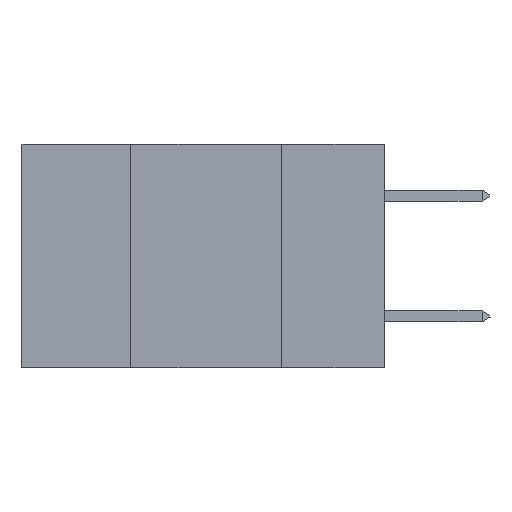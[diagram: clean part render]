
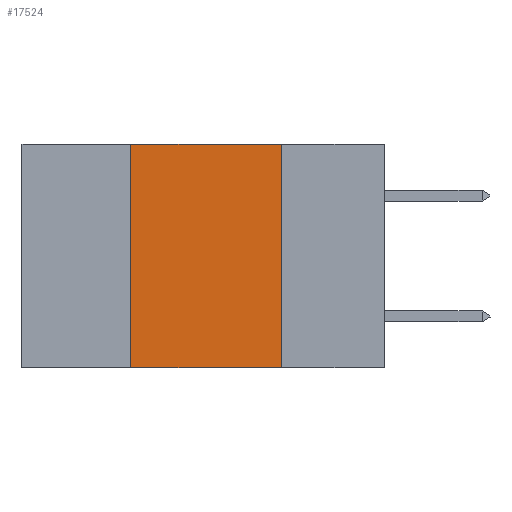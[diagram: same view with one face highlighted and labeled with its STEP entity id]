
A CAD part, left-side view. The second image highlights one B-rep face of the part: STEP entity #17524.
In plain terms, the highlighted planar face has unit normal (-1, 0, 0).
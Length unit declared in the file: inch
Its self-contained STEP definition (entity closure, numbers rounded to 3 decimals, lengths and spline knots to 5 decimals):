
#1654 = DIRECTION ( 'NONE',  ( 0., -1., 0. ) ) ;
#2041 = LINE ( 'NONE', #10031, #15891 ) ;
#3149 = LINE ( 'NONE', #19741, #7271 ) ;
#3609 = FACE_OUTER_BOUND ( 'NONE', #18241, .T. ) ;
#3723 = ORIENTED_EDGE ( 'NONE', *, *, #15651, .F. ) ;
#3820 = DIRECTION ( 'NONE',  ( 1., 0., 0. ) ) ;
#7271 = VECTOR ( 'NONE', #19822, 39.37008 ) ;
#7329 = ORIENTED_EDGE ( 'NONE', *, *, #17406, .F. ) ;
#7389 = EDGE_CURVE ( 'NONE', #21103, #18453, #3149, .T. ) ;
#7455 = ORIENTED_EDGE ( 'NONE', *, *, #13287, .F. ) ;
#8096 = CARTESIAN_POINT ( 'NONE',  ( 0., 0.17, 0. ) ) ;
#9684 = LINE ( 'NONE', #21087, #15256 ) ;
#10031 = CARTESIAN_POINT ( 'NONE',  ( 0., 0.42, 0. ) ) ;
#10221 = CARTESIAN_POINT ( 'NONE',  ( 0., 0.42, -0.37 ) ) ;
#10476 = DIRECTION ( 'NONE',  ( 0., 0., -1. ) ) ;
#10806 = AXIS2_PLACEMENT_3D ( 'NONE', #21376, #3820, #14563 ) ;
#12486 = LINE ( 'NONE', #15685, #18281 ) ;
#13287 = EDGE_CURVE ( 'NONE', #14490, #18453, #12486, .T. ) ;
#13511 = CARTESIAN_POINT ( 'NONE',  ( 0., 0.17, -0.37 ) ) ;
#14490 = VERTEX_POINT ( 'NONE', #8096 ) ;
#14563 = DIRECTION ( 'NONE',  ( 0., 0., -1. ) ) ;
#14813 = ORIENTED_EDGE ( 'NONE', *, *, #7389, .T. ) ;
#15256 = VECTOR ( 'NONE', #1654, 39.37008 ) ;
#15651 = EDGE_CURVE ( 'NONE', #21103, #16280, #2041, .T. ) ;
#15685 = CARTESIAN_POINT ( 'NONE',  ( 0., 0.17, 0. ) ) ;
#15891 = VECTOR ( 'NONE', #19124, 39.37008 ) ;
#16280 = VERTEX_POINT ( 'NONE', #17961 ) ;
#17406 = EDGE_CURVE ( 'NONE', #16280, #14490, #9684, .T. ) ;
#17524 = ADVANCED_FACE ( 'NONE', ( #3609 ), #19687, .F. ) ;
#17961 = CARTESIAN_POINT ( 'NONE',  ( 0., 0.42, 0. ) ) ;
#18241 = EDGE_LOOP ( 'NONE', ( #7455, #7329, #3723, #14813 ) ) ;
#18281 = VECTOR ( 'NONE', #10476, 39.37008 ) ;
#18453 = VERTEX_POINT ( 'NONE', #13511 ) ;
#19124 = DIRECTION ( 'NONE',  ( 0., 0., 1. ) ) ;
#19687 = PLANE ( 'NONE',  #10806 ) ;
#19741 = CARTESIAN_POINT ( 'NONE',  ( 0., 0.6, -0.37 ) ) ;
#19822 = DIRECTION ( 'NONE',  ( 0., -1., 0. ) ) ;
#21087 = CARTESIAN_POINT ( 'NONE',  ( 0., 0.6, 0. ) ) ;
#21103 = VERTEX_POINT ( 'NONE', #10221 ) ;
#21376 = CARTESIAN_POINT ( 'NONE',  ( 0., 0.6, 0. ) ) ;
